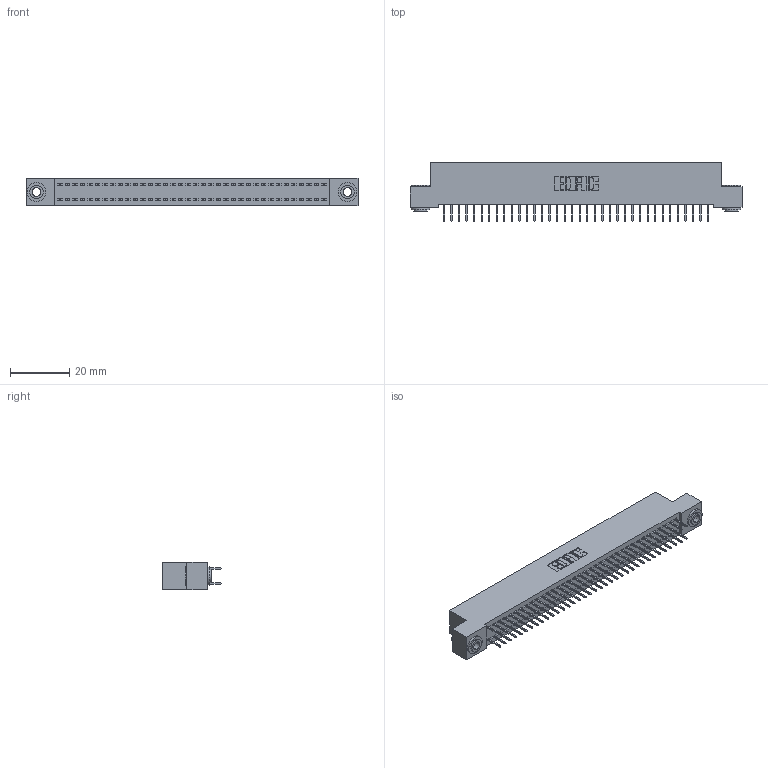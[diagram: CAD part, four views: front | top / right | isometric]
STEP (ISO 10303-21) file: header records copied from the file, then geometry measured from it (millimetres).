
FILE_DESCRIPTION (( 'STEP AP203' ), '1' );
FILE_NAME ('342-072-524-203.STEP', '2018-08-13T10:09:13', ( '' ), ( '' ), 'SwSTEP 2.0', 'SolidWorks 2016', '' );
FILE_SCHEMA (( 'CONFIG_CONTROL_DESIGN' ));
Length unit declared in the file: inch
Products named in the file (4): 342 Part_.156 TH; 345-292-001_345-293-124; 342-250-002_345-250-002-102; 342-072-524-203
Assembly tree (75 placements, depth 2):
  342-072-524-203
    342 Part_.156 TH
    345-292-001_345-293-124  x72
    342-250-002_345-250-002-102  x2
Bounding box: 111.76 x 19.69 x 9.4 mm (x, y, z)
Volume: 9927.1 mm3; surface area: 15941.6 mm2
Topology: 75 solids, 75 shells, 4180 faces, 11823 edges, 7590 vertices
Faces by surface type: plane 3100, cylinder 1072, cone 8
Entity records: 24528 total; most frequent: CARTESIAN_POINT 4045, ORIENTED_EDGE 3974, DIRECTION 3501, EDGE_CURVE 1987, VECTOR 1839, LINE 1839, VERTEX_POINT 1318, AXIS2_PLACEMENT_3D 831
